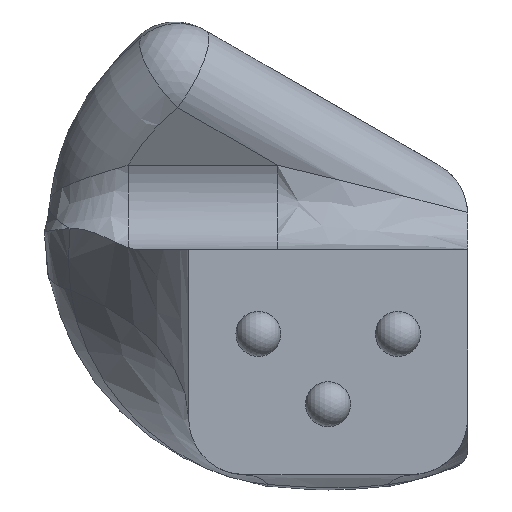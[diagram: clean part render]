
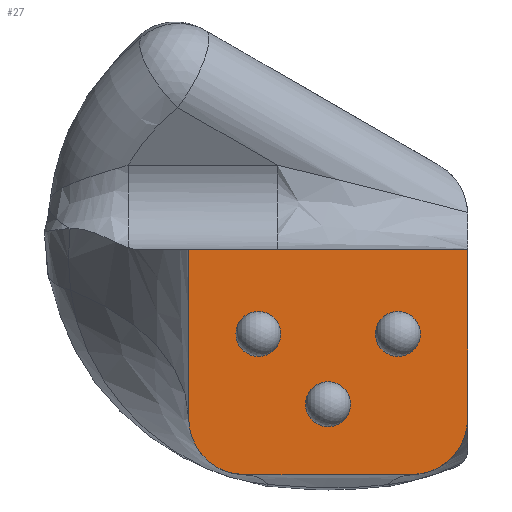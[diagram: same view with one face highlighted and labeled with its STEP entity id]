
A CAD part, left-side view. The second image highlights one B-rep face of the part: STEP entity #27.
In plain terms, the highlighted planar face has unit normal (-1, 0, 0).
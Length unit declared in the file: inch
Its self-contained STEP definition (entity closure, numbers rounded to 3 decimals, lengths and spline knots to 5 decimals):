
#14 = VERTEX_POINT ( 'NONE', #862 ) ;
#16 = VERTEX_POINT ( 'NONE', #693 ) ;
#27 = ADVANCED_FACE ( 'NONE', ( #1462, #1466, #1452, #1438 ), #1013, .F. ) ;
#42 = ORIENTED_EDGE ( 'NONE', *, *, #1382, .F. ) ;
#49 = CARTESIAN_POINT ( 'NONE',  ( 8.48393, 0.48819, 0.24606 ) ) ;
#108 = CARTESIAN_POINT ( 'NONE',  ( 8.48393, 0.19685, 0.19685 ) ) ;
#138 = DIRECTION ( 'NONE',  ( -1., 0., 0. ) ) ;
#164 = AXIS2_PLACEMENT_3D ( 'NONE', #49, #931, #197 ) ;
#189 = CARTESIAN_POINT ( 'NONE',  ( 8.48393, 0.97638, 0.19685 ) ) ;
#197 = DIRECTION ( 'NONE',  ( 0., 0., -1. ) ) ;
#198 = ORIENTED_EDGE ( 'NONE', *, *, #1675, .T. ) ;
#204 = DIRECTION ( 'NONE',  ( 0., 0., -1. ) ) ;
#250 = CARTESIAN_POINT ( 'NONE',  ( 8.48393, 0.48819, 0. ) ) ;
#253 = DIRECTION ( 'NONE',  ( 0., 0., -1. ) ) ;
#275 = DIRECTION ( 'NONE',  ( -1., 0., 0. ) ) ;
#320 = DIRECTION ( 'NONE',  ( -1., 0., 0. ) ) ;
#327 = ORIENTED_EDGE ( 'NONE', *, *, #1569, .T. ) ;
#335 = AXIS2_PLACEMENT_3D ( 'NONE', #1059, #320, #1196 ) ;
#341 = VERTEX_POINT ( 'NONE', #1578 ) ;
#364 = AXIS2_PLACEMENT_3D ( 'NONE', #1017, #275, #1154 ) ;
#399 = ORIENTED_EDGE ( 'NONE', *, *, #1398, .T. ) ;
#407 = VERTEX_POINT ( 'NONE', #189 ) ;
#433 = AXIS2_PLACEMENT_3D ( 'NONE', #108, #989, #253 ) ;
#460 = EDGE_LOOP ( 'NONE', ( #497 ) ) ;
#497 = ORIENTED_EDGE ( 'NONE', *, *, #1429, .F. ) ;
#504 = CARTESIAN_POINT ( 'NONE',  ( 8.48393, 0., 8.44049 ) ) ;
#561 = ORIENTED_EDGE ( 'NONE', *, *, #1444, .F. ) ;
#647 = CARTESIAN_POINT ( 'NONE',  ( 8.48393, 0.73228, 0.41339 ) ) ;
#658 = VERTEX_POINT ( 'NONE', #720 ) ;
#667 = ORIENTED_EDGE ( 'NONE', *, *, #1419, .T. ) ;
#693 = CARTESIAN_POINT ( 'NONE',  ( 8.48393, 0., 0.19685 ) ) ;
#720 = CARTESIAN_POINT ( 'NONE',  ( 8.48393, 0.97638, 0.7874 ) ) ;
#723 = ORIENTED_EDGE ( 'NONE', *, *, #1522, .F. ) ;
#777 = CARTESIAN_POINT ( 'NONE',  ( 8.48393, 0.48819, 0.16732 ) ) ;
#826 = VERTEX_POINT ( 'NONE', #777 ) ;
#828 = VERTEX_POINT ( 'NONE', #1319 ) ;
#844 = VERTEX_POINT ( 'NONE', #647 ) ;
#856 = CIRCLE ( 'NONE', #1181, 0.19685 ) ;
#862 = CARTESIAN_POINT ( 'NONE',  ( 8.48393, 0., 0.7874 ) ) ;
#872 = VECTOR ( 'NONE', #204, 39.37008 ) ;
#873 = CARTESIAN_POINT ( 'NONE',  ( 8.48393, 0.77953, 0.19685 ) ) ;
#888 = LINE ( 'NONE', #1362, #872 ) ;
#898 = CIRCLE ( 'NONE', #164, 0.07874 ) ;
#900 = DIRECTION ( 'NONE',  ( 1., 0., 0. ) ) ;
#931 = DIRECTION ( 'NONE',  ( -1., 0., 0. ) ) ;
#955 = CIRCLE ( 'NONE', #335, 0.07874 ) ;
#957 = CIRCLE ( 'NONE', #364, 0.07874 ) ;
#974 = LINE ( 'NONE', #504, #980 ) ;
#979 = CIRCLE ( 'NONE', #433, 0.19685 ) ;
#980 = VECTOR ( 'NONE', #1272, 39.37008 ) ;
#981 = VECTOR ( 'NONE', #984, 39.37008 ) ;
#984 = DIRECTION ( 'NONE',  ( 0., -1., 0. ) ) ;
#989 = DIRECTION ( 'NONE',  ( -1., 0., 0. ) ) ;
#997 = DIRECTION ( 'NONE',  ( 0., 0., -1. ) ) ;
#998 = LINE ( 'NONE', #250, #981 ) ;
#1003 = VECTOR ( 'NONE', #1113, 39.37008 ) ;
#1005 = LINE ( 'NONE', #1673, #1003 ) ;
#1013 = PLANE ( 'NONE',  #1328 ) ;
#1016 = CARTESIAN_POINT ( 'NONE',  ( 8.48393, 2.82639, 11.34684 ) ) ;
#1017 = CARTESIAN_POINT ( 'NONE',  ( 8.48393, 0.73228, 0.49213 ) ) ;
#1022 = DIRECTION ( 'NONE',  ( 0., 0., -1. ) ) ;
#1059 = CARTESIAN_POINT ( 'NONE',  ( 8.48393, 0.24409, 0.49213 ) ) ;
#1113 = DIRECTION ( 'NONE',  ( 0., -1., 0. ) ) ;
#1154 = DIRECTION ( 'NONE',  ( 0., 0., -1. ) ) ;
#1178 = CARTESIAN_POINT ( 'NONE',  ( 8.48393, 0.19685, 0. ) ) ;
#1181 = AXIS2_PLACEMENT_3D ( 'NONE', #873, #138, #1022 ) ;
#1196 = DIRECTION ( 'NONE',  ( 0., 0., -1. ) ) ;
#1272 = DIRECTION ( 'NONE',  ( 0., 0., 1. ) ) ;
#1319 = CARTESIAN_POINT ( 'NONE',  ( 8.48393, 0.24409, 0.41339 ) ) ;
#1328 = AXIS2_PLACEMENT_3D ( 'NONE', #1016, #900, #997 ) ;
#1333 = ORIENTED_EDGE ( 'NONE', *, *, #1407, .T. ) ;
#1362 = CARTESIAN_POINT ( 'NONE',  ( 8.48393, 0.97638, 8.44049 ) ) ;
#1373 = EDGE_LOOP ( 'NONE', ( #42, #327, #198, #399, #1333, #667 ) ) ;
#1382 = EDGE_CURVE ( 'NONE', #658, #14, #1005, .T. ) ;
#1398 = EDGE_CURVE ( 'NONE', #341, #1708, #998, .T. ) ;
#1407 = EDGE_CURVE ( 'NONE', #1708, #16, #979, .T. ) ;
#1419 = EDGE_CURVE ( 'NONE', #16, #14, #974, .T. ) ;
#1429 = EDGE_CURVE ( 'NONE', #844, #844, #957, .T. ) ;
#1438 = FACE_BOUND ( 'NONE', #1649, .T. ) ;
#1444 = EDGE_CURVE ( 'NONE', #828, #828, #955, .T. ) ;
#1452 = FACE_BOUND ( 'NONE', #460, .T. ) ;
#1462 = FACE_BOUND ( 'NONE', #1678, .T. ) ;
#1466 = FACE_OUTER_BOUND ( 'NONE', #1373, .T. ) ;
#1522 = EDGE_CURVE ( 'NONE', #826, #826, #898, .T. ) ;
#1569 = EDGE_CURVE ( 'NONE', #658, #407, #888, .T. ) ;
#1578 = CARTESIAN_POINT ( 'NONE',  ( 8.48393, 0.77953, 0. ) ) ;
#1649 = EDGE_LOOP ( 'NONE', ( #561 ) ) ;
#1673 = CARTESIAN_POINT ( 'NONE',  ( 8.48393, 0.48819, 0.7874 ) ) ;
#1675 = EDGE_CURVE ( 'NONE', #407, #341, #856, .T. ) ;
#1678 = EDGE_LOOP ( 'NONE', ( #723 ) ) ;
#1708 = VERTEX_POINT ( 'NONE', #1178 ) ;
